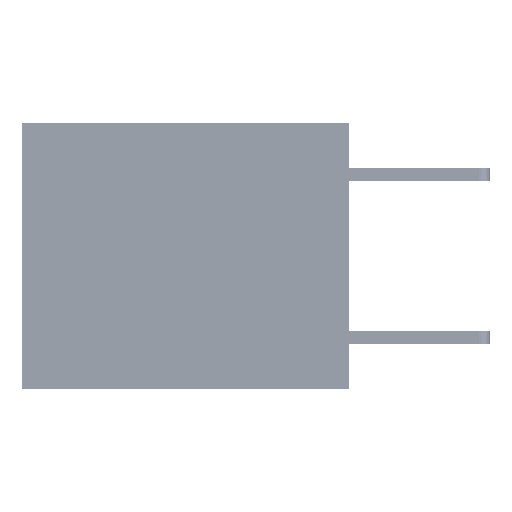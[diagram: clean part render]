
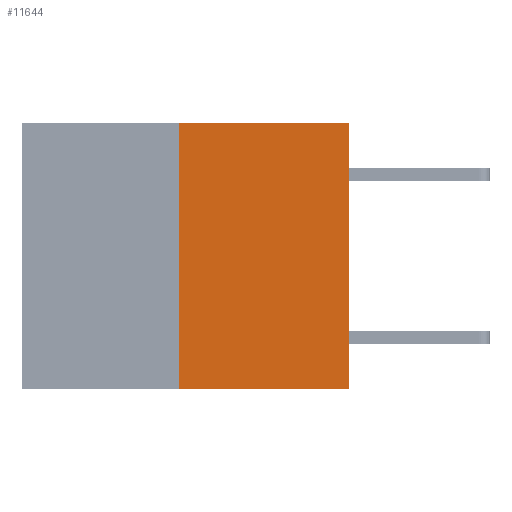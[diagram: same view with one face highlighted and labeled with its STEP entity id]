
A CAD part, left-side view. The second image highlights one B-rep face of the part: STEP entity #11644.
In plain terms, the highlighted planar face has unit normal (-1, 0, 0).
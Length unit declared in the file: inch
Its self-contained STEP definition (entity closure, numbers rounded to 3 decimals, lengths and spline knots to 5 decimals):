
#323 = CARTESIAN_POINT ( 'NONE',  ( 0., 0., 0. ) ) ;
#769 = CARTESIAN_POINT ( 'NONE',  ( 0., 0., -0.49 ) ) ;
#1742 = ORIENTED_EDGE ( 'NONE', *, *, #9452, .T. ) ;
#1947 = FACE_OUTER_BOUND ( 'NONE', #32672, .T. ) ;
#4999 = DIRECTION ( 'NONE',  ( 1., 0., 0. ) ) ;
#5935 = DIRECTION ( 'NONE',  ( 0., -1., 0. ) ) ;
#6450 = EDGE_CURVE ( 'NONE', #29510, #13098, #10890, .T. ) ;
#6780 = VECTOR ( 'NONE', #5935, 39.37008 ) ;
#7260 = DIRECTION ( 'NONE',  ( 0., 0., -1. ) ) ;
#9452 = EDGE_CURVE ( 'NONE', #30529, #29510, #23036, .T. ) ;
#10890 = LINE ( 'NONE', #323, #24978 ) ;
#11644 = ADVANCED_FACE ( 'NONE', ( #1947 ), #33050, .F. ) ;
#12020 = EDGE_CURVE ( 'NONE', #30529, #26341, #20848, .T. ) ;
#13098 = VERTEX_POINT ( 'NONE', #18479 ) ;
#13327 = VECTOR ( 'NONE', #13487, 39.37008 ) ;
#13487 = DIRECTION ( 'NONE',  ( 0., 0., 1. ) ) ;
#13876 = CARTESIAN_POINT ( 'NONE',  ( 0., 0.6, -0.49 ) ) ;
#15133 = DIRECTION ( 'NONE',  ( 0., -1., 0. ) ) ;
#16696 = CARTESIAN_POINT ( 'NONE',  ( 0., 0.312, -0.49 ) ) ;
#16803 = LINE ( 'NONE', #26140, #23444 ) ;
#18479 = CARTESIAN_POINT ( 'NONE',  ( 0., 0., 0. ) ) ;
#19118 = ORIENTED_EDGE ( 'NONE', *, *, #30229, .F. ) ;
#20629 = AXIS2_PLACEMENT_3D ( 'NONE', #35874, #4999, #7260 ) ;
#20848 = LINE ( 'NONE', #30377, #13327 ) ;
#23036 = LINE ( 'NONE', #13876, #6780 ) ;
#23444 = VECTOR ( 'NONE', #15133, 39.37008 ) ;
#24978 = VECTOR ( 'NONE', #25865, 39.37008 ) ;
#25865 = DIRECTION ( 'NONE',  ( 0., 0., 1. ) ) ;
#26140 = CARTESIAN_POINT ( 'NONE',  ( 0., 0.6, 0. ) ) ;
#26228 = ORIENTED_EDGE ( 'NONE', *, *, #12020, .F. ) ;
#26341 = VERTEX_POINT ( 'NONE', #32473 ) ;
#26820 = ORIENTED_EDGE ( 'NONE', *, *, #6450, .T. ) ;
#29510 = VERTEX_POINT ( 'NONE', #769 ) ;
#30229 = EDGE_CURVE ( 'NONE', #26341, #13098, #16803, .T. ) ;
#30377 = CARTESIAN_POINT ( 'NONE',  ( 0., 0.312, -0.49 ) ) ;
#30529 = VERTEX_POINT ( 'NONE', #16696 ) ;
#32473 = CARTESIAN_POINT ( 'NONE',  ( 0., 0.312, 0. ) ) ;
#32672 = EDGE_LOOP ( 'NONE', ( #26228, #1742, #26820, #19118 ) ) ;
#33050 = PLANE ( 'NONE',  #20629 ) ;
#35874 = CARTESIAN_POINT ( 'NONE',  ( 0., 0.6, 0. ) ) ;
